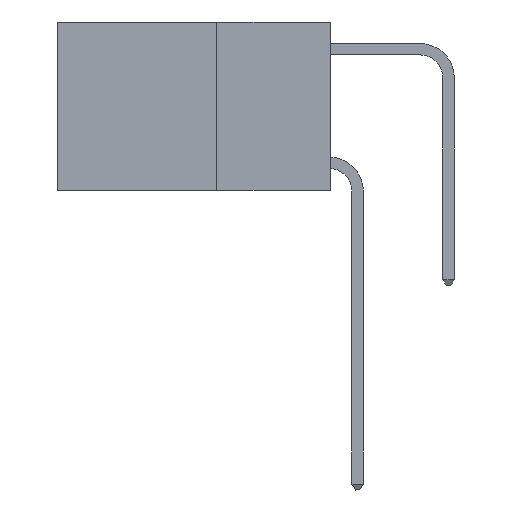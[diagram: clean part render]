
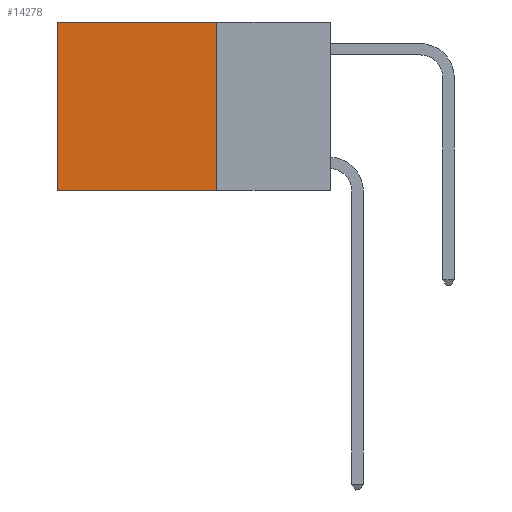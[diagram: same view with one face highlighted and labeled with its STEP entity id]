
A CAD part, left-side view. The second image highlights one B-rep face of the part: STEP entity #14278.
In plain terms, the highlighted planar face has unit normal (-1, 0, 0).
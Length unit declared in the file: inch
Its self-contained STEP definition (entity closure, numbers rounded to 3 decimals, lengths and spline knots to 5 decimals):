
#492 = VERTEX_POINT ( 'NONE', #16429 ) ;
#1017 = VERTEX_POINT ( 'NONE', #11277 ) ;
#1368 = DIRECTION ( 'NONE',  ( 0., 0., -1. ) ) ;
#2336 = LINE ( 'NONE', #6834, #17381 ) ;
#2640 = EDGE_CURVE ( 'NONE', #6650, #492, #8780, .T. ) ;
#3463 = FACE_OUTER_BOUND ( 'NONE', #9729, .T. ) ;
#3526 = CARTESIAN_POINT ( 'NONE',  ( 0.2625, 0.25, -0.37 ) ) ;
#4289 = VECTOR ( 'NONE', #1368, 39.37008 ) ;
#5732 = ORIENTED_EDGE ( 'NONE', *, *, #13517, .F. ) ;
#6052 = CARTESIAN_POINT ( 'NONE',  ( 0.2625, 0.25, 0. ) ) ;
#6370 = VERTEX_POINT ( 'NONE', #3526 ) ;
#6496 = PLANE ( 'NONE',  #18671 ) ;
#6650 = VERTEX_POINT ( 'NONE', #6052 ) ;
#6834 = CARTESIAN_POINT ( 'NONE',  ( 0.2625, 0.25, 0. ) ) ;
#7617 = CARTESIAN_POINT ( 'NONE',  ( 0.2625, 0.25, 0. ) ) ;
#8780 = LINE ( 'NONE', #7617, #19058 ) ;
#8798 = LINE ( 'NONE', #11511, #4289 ) ;
#9026 = VECTOR ( 'NONE', #12825, 39.37008 ) ;
#9729 = EDGE_LOOP ( 'NONE', ( #18986, #5732, #10371, #18026 ) ) ;
#10124 = CARTESIAN_POINT ( 'NONE',  ( 0.2625, 0.25, -0.37 ) ) ;
#10371 = ORIENTED_EDGE ( 'NONE', *, *, #12347, .F. ) ;
#10727 = EDGE_CURVE ( 'NONE', #492, #1017, #8798, .T. ) ;
#10953 = DIRECTION ( 'NONE',  ( 1., 0., 0. ) ) ;
#11277 = CARTESIAN_POINT ( 'NONE',  ( 0.2625, 0.6, -0.37 ) ) ;
#11511 = CARTESIAN_POINT ( 'NONE',  ( 0.2625, 0.6, 0. ) ) ;
#12217 = DIRECTION ( 'NONE',  ( 0., 0., -1. ) ) ;
#12347 = EDGE_CURVE ( 'NONE', #6650, #6370, #2336, .T. ) ;
#12825 = DIRECTION ( 'NONE',  ( 0., 1., 0. ) ) ;
#13444 = DIRECTION ( 'NONE',  ( 0., 1., 0. ) ) ;
#13517 = EDGE_CURVE ( 'NONE', #6370, #1017, #17233, .T. ) ;
#14278 = ADVANCED_FACE ( 'NONE', ( #3463 ), #6496, .F. ) ;
#16429 = CARTESIAN_POINT ( 'NONE',  ( 0.2625, 0.6, 0. ) ) ;
#17233 = LINE ( 'NONE', #10124, #9026 ) ;
#17381 = VECTOR ( 'NONE', #18796, 39.37008 ) ;
#18026 = ORIENTED_EDGE ( 'NONE', *, *, #2640, .T. ) ;
#18263 = CARTESIAN_POINT ( 'NONE',  ( 0.2625, 0.25, 0. ) ) ;
#18671 = AXIS2_PLACEMENT_3D ( 'NONE', #18263, #10953, #12217 ) ;
#18796 = DIRECTION ( 'NONE',  ( 0., 0., -1. ) ) ;
#18986 = ORIENTED_EDGE ( 'NONE', *, *, #10727, .T. ) ;
#19058 = VECTOR ( 'NONE', #13444, 39.37008 ) ;
